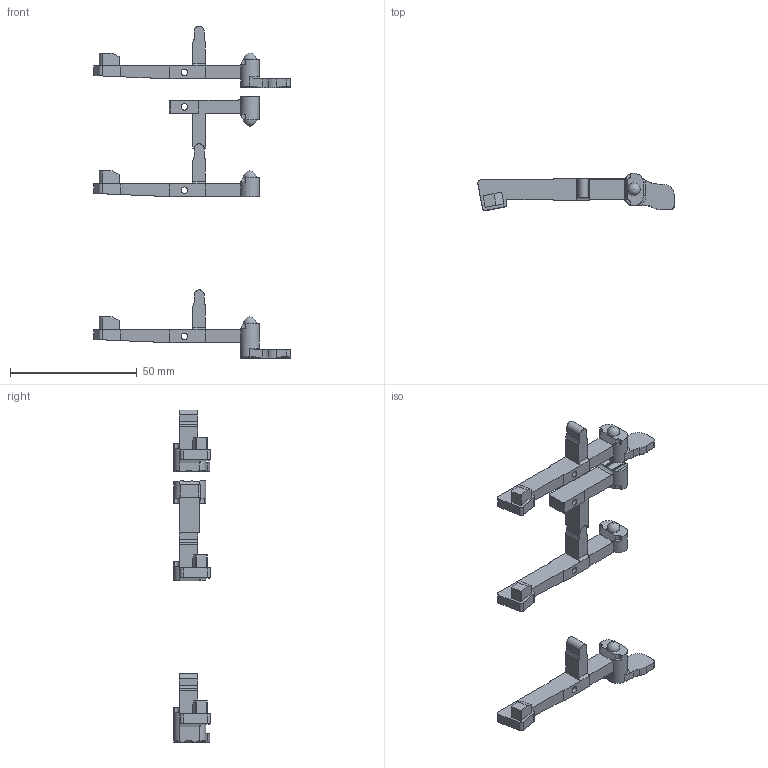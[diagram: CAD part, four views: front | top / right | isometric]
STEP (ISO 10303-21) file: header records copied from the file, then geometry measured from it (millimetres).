
FILE_DESCRIPTION(/* description */ (''),/* implementation_level */ '2;1');
FILE_NAME(/* name */ '9mm Mag Catch Levers.step',/* time_stamp */ '2020-02-15T23:57:20-06:00',/* author */ (''),/* organization */ (''),/* preprocessor_version */ 'ST-DEVELOPER v18',/* originating_system */ 'Autodesk Translation Framework v8.12.0.6',/* authorisation */ '');
FILE_SCHEMA (('AUTOMOTIVE_DESIGN { 1 0 10303 214 3 1 1 }'));
Length unit declared in the file: inch
Products named in the file (1): VAR9 Mod 2
Bounding box: 77.48 x 14.56 x 131.03 mm (x, y, z)
Volume: 14638.4 mm3; surface area: 10091.7 mm2
Topology: 4 solids, 4 shells, 252 faces, 713 edges, 472 vertices
Faces by surface type: plane 136, cylinder 108, torus 4, sphere 4
Full cylindrical faces by diameter (mm): 2.54 x4
Entity records: 8411 total; most frequent: CARTESIAN_POINT 1653, DIRECTION 1432, ORIENTED_EDGE 1418, EDGE_CURVE 709, AXIS2_PLACEMENT_3D 507, VERTEX_POINT 472, LINE 418, VECTOR 418
